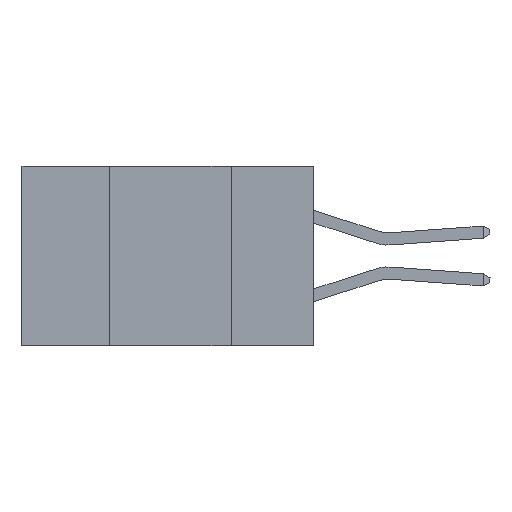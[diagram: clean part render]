
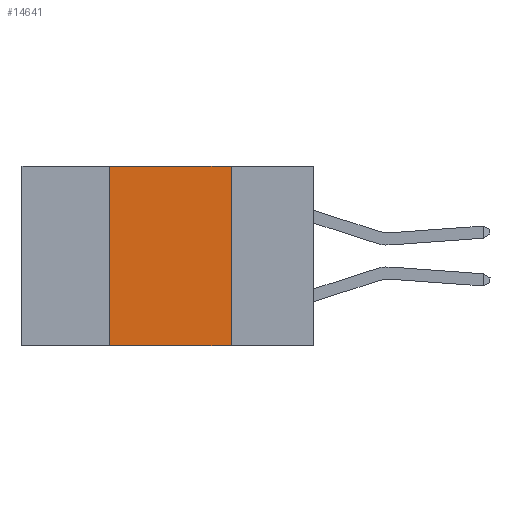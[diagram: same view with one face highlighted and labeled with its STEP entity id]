
A CAD part, left-side view. The second image highlights one B-rep face of the part: STEP entity #14641.
In plain terms, the highlighted planar face has unit normal (-1, 0, 0).
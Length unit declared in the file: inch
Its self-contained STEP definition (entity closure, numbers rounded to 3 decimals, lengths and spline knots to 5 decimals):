
#1613 = VECTOR ( 'NONE', #16495, 39.37008 ) ;
#1834 = CARTESIAN_POINT ( 'NONE',  ( 0., 0.6, -0.37 ) ) ;
#3303 = CARTESIAN_POINT ( 'NONE',  ( 0., 0.17, -0.37 ) ) ;
#4717 = EDGE_CURVE ( 'NONE', #23625, #18809, #35356, .T. ) ;
#6500 = VECTOR ( 'NONE', #25417, 39.37008 ) ;
#6691 = DIRECTION ( 'NONE',  ( 1., 0., 0. ) ) ;
#7466 = VECTOR ( 'NONE', #11701, 39.37008 ) ;
#9745 = CARTESIAN_POINT ( 'NONE',  ( 0., 0.6, 0. ) ) ;
#10040 = VECTOR ( 'NONE', #25729, 39.37008 ) ;
#11701 = DIRECTION ( 'NONE',  ( 0., 0., -1. ) ) ;
#14641 = ADVANCED_FACE ( 'NONE', ( #31407 ), #29211, .F. ) ;
#15256 = EDGE_CURVE ( 'NONE', #23625, #30782, #20384, .T. ) ;
#16495 = DIRECTION ( 'NONE',  ( 0., -1., 0. ) ) ;
#17455 = ORIENTED_EDGE ( 'NONE', *, *, #15256, .F. ) ;
#18809 = VERTEX_POINT ( 'NONE', #3303 ) ;
#19816 = CARTESIAN_POINT ( 'NONE',  ( 0., 0.42, -0.37 ) ) ;
#20202 = CARTESIAN_POINT ( 'NONE',  ( 0., 0.42, 0. ) ) ;
#20384 = LINE ( 'NONE', #31362, #10040 ) ;
#20991 = DIRECTION ( 'NONE',  ( 0., 0., -1. ) ) ;
#21986 = EDGE_LOOP ( 'NONE', ( #26747, #25688, #17455, #27144 ) ) ;
#23113 = EDGE_CURVE ( 'NONE', #28419, #18809, #32459, .T. ) ;
#23625 = VERTEX_POINT ( 'NONE', #19816 ) ;
#25417 = DIRECTION ( 'NONE',  ( 0., -1., 0. ) ) ;
#25688 = ORIENTED_EDGE ( 'NONE', *, *, #28392, .F. ) ;
#25729 = DIRECTION ( 'NONE',  ( 0., 0., 1. ) ) ;
#26747 = ORIENTED_EDGE ( 'NONE', *, *, #23113, .F. ) ;
#27144 = ORIENTED_EDGE ( 'NONE', *, *, #4717, .T. ) ;
#27681 = CARTESIAN_POINT ( 'NONE',  ( 0., 0.17, 0. ) ) ;
#27976 = CARTESIAN_POINT ( 'NONE',  ( 0., 0.6, 0. ) ) ;
#28392 = EDGE_CURVE ( 'NONE', #30782, #28419, #35431, .T. ) ;
#28419 = VERTEX_POINT ( 'NONE', #33906 ) ;
#29211 = PLANE ( 'NONE',  #34373 ) ;
#30782 = VERTEX_POINT ( 'NONE', #20202 ) ;
#31362 = CARTESIAN_POINT ( 'NONE',  ( 0., 0.42, 0. ) ) ;
#31407 = FACE_OUTER_BOUND ( 'NONE', #21986, .T. ) ;
#32459 = LINE ( 'NONE', #27681, #7466 ) ;
#33906 = CARTESIAN_POINT ( 'NONE',  ( 0., 0.17, 0. ) ) ;
#34373 = AXIS2_PLACEMENT_3D ( 'NONE', #9745, #6691, #20991 ) ;
#35356 = LINE ( 'NONE', #1834, #1613 ) ;
#35431 = LINE ( 'NONE', #27976, #6500 ) ;
